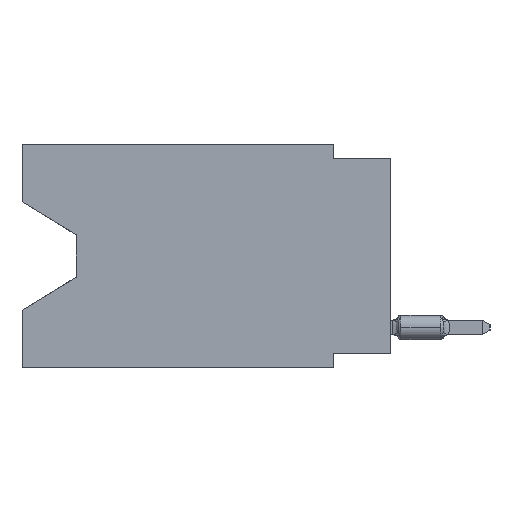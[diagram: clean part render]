
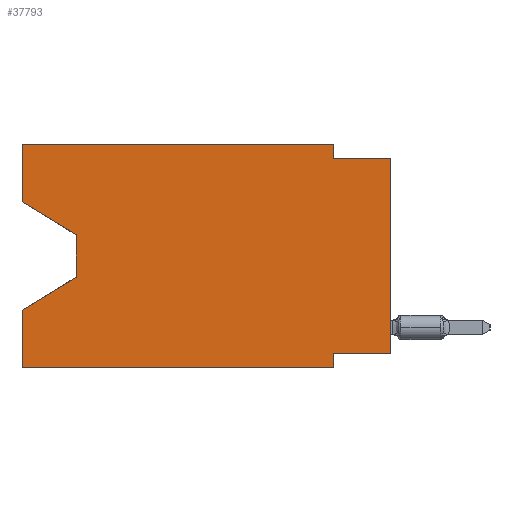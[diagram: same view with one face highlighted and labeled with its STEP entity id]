
A CAD part, left-side view. The second image highlights one B-rep face of the part: STEP entity #37793.
In plain terms, the highlighted planar face has unit normal (-1, 0, 0).
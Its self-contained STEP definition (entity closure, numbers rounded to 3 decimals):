
#69 = VERTEX_POINT ( 'NONE', #26142 ) ;
#154 = ORIENTED_EDGE ( 'NONE', *, *, #14962, .F. ) ;
#1042 = VERTEX_POINT ( 'NONE', #56922 ) ;
#2557 = DIRECTION ( 'NONE',  ( 0., 0.855, -0.519 ) ) ;
#2766 = VECTOR ( 'NONE', #8453, 1000. ) ;
#2847 = DIRECTION ( 'NONE',  ( 0., -1., 0. ) ) ;
#4312 = VERTEX_POINT ( 'NONE', #74643 ) ;
#6569 = LINE ( 'NONE', #58709, #25893 ) ;
#6645 = LINE ( 'NONE', #53426, #15274 ) ;
#7734 = DIRECTION ( 'NONE',  ( 0., 0., -1. ) ) ;
#8318 = LINE ( 'NONE', #25927, #33434 ) ;
#8453 = DIRECTION ( 'NONE',  ( 0., 0., -1. ) ) ;
#9292 = ORIENTED_EDGE ( 'NONE', *, *, #17592, .T. ) ;
#9833 = CARTESIAN_POINT ( 'NONE',  ( 0., 2.54, -9.906 ) ) ;
#10333 = LINE ( 'NONE', #52889, #56960 ) ;
#10784 = CARTESIAN_POINT ( 'NONE',  ( 0., 2.54, 0. ) ) ;
#10847 = CARTESIAN_POINT ( 'NONE',  ( 0., 2.54, 0. ) ) ;
#12962 = DIRECTION ( 'NONE',  ( 0., 0., -1. ) ) ;
#13139 = DIRECTION ( 'NONE',  ( 0., 0., -1. ) ) ;
#13227 = CARTESIAN_POINT ( 'NONE',  ( 0., 13.97, -4.013 ) ) ;
#14686 = AXIS2_PLACEMENT_3D ( 'NONE', #66761, #37614, #13139 ) ;
#14962 = EDGE_CURVE ( 'NONE', #1042, #27319, #39670, .T. ) ;
#15274 = VECTOR ( 'NONE', #18509, 1000. ) ;
#17400 = CARTESIAN_POINT ( 'NONE',  ( 0., 16.383, -2.546 ) ) ;
#17592 = EDGE_CURVE ( 'NONE', #47912, #22956, #18839, .T. ) ;
#18509 = DIRECTION ( 'NONE',  ( 0., 1., 0. ) ) ;
#18839 = LINE ( 'NONE', #60257, #19649 ) ;
#19649 = VECTOR ( 'NONE', #7734, 1000. ) ;
#20201 = ORIENTED_EDGE ( 'NONE', *, *, #43544, .F. ) ;
#20204 = EDGE_CURVE ( 'NONE', #65862, #1042, #6569, .T. ) ;
#20743 = FACE_OUTER_BOUND ( 'NONE', #42780, .T. ) ;
#22283 = DIRECTION ( 'NONE',  ( 0., 0., 1. ) ) ;
#22810 = VERTEX_POINT ( 'NONE', #56799 ) ;
#22956 = VERTEX_POINT ( 'NONE', #27642 ) ;
#23275 = ORIENTED_EDGE ( 'NONE', *, *, #66403, .F. ) ;
#23717 = EDGE_CURVE ( 'NONE', #22956, #34299, #8318, .T. ) ;
#25504 = VECTOR ( 'NONE', #57700, 1000. ) ;
#25619 = EDGE_CURVE ( 'NONE', #22810, #41762, #6645, .T. ) ;
#25893 = VECTOR ( 'NONE', #22283, 1000. ) ;
#25927 = CARTESIAN_POINT ( 'NONE',  ( 0., 13.97, -5.893 ) ) ;
#26142 = CARTESIAN_POINT ( 'NONE',  ( 0., 0., -0.635 ) ) ;
#26453 = CARTESIAN_POINT ( 'NONE',  ( 0., 2.54, -9.906 ) ) ;
#27319 = VERTEX_POINT ( 'NONE', #10847 ) ;
#27642 = CARTESIAN_POINT ( 'NONE',  ( 0., 13.97, -5.893 ) ) ;
#28023 = ORIENTED_EDGE ( 'NONE', *, *, #20204, .F. ) ;
#28178 = LINE ( 'NONE', #33178, #43076 ) ;
#28193 = VECTOR ( 'NONE', #28244, 1000. ) ;
#28244 = DIRECTION ( 'NONE',  ( 0., -0.855, -0.519 ) ) ;
#29385 = CARTESIAN_POINT ( 'NONE',  ( 0., 16.383, -2.546 ) ) ;
#30999 = VERTEX_POINT ( 'NONE', #74027 ) ;
#32113 = ORIENTED_EDGE ( 'NONE', *, *, #50423, .T. ) ;
#32631 = DIRECTION ( 'NONE',  ( 0., 0., 1. ) ) ;
#33057 = VERTEX_POINT ( 'NONE', #9833 ) ;
#33178 = CARTESIAN_POINT ( 'NONE',  ( 0., 16.383, -9.906 ) ) ;
#33434 = VECTOR ( 'NONE', #2557, 1000. ) ;
#33572 = VECTOR ( 'NONE', #12962, 1000. ) ;
#34106 = ORIENTED_EDGE ( 'NONE', *, *, #59403, .F. ) ;
#34299 = VERTEX_POINT ( 'NONE', #51605 ) ;
#34538 = LINE ( 'NONE', #10784, #33572 ) ;
#34739 = LINE ( 'NONE', #29385, #28193 ) ;
#36752 = EDGE_CURVE ( 'NONE', #4312, #34299, #61768, .T. ) ;
#37614 = DIRECTION ( 'NONE',  ( 1., 0., 0. ) ) ;
#37793 = ADVANCED_FACE ( 'NONE', ( #20743 ), #44136, .F. ) ;
#39302 = DIRECTION ( 'NONE',  ( 0., -1., 0. ) ) ;
#39670 = LINE ( 'NONE', #75320, #25504 ) ;
#41762 = VERTEX_POINT ( 'NONE', #55363 ) ;
#42780 = EDGE_LOOP ( 'NONE', ( #43216, #9292, #49295, #65210, #62398, #23275, #44096, #32113, #34106, #20201, #154, #28023 ) ) ;
#43076 = VECTOR ( 'NONE', #39302, 1000. ) ;
#43216 = ORIENTED_EDGE ( 'NONE', *, *, #65258, .T. ) ;
#43544 = EDGE_CURVE ( 'NONE', #27319, #30999, #34538, .T. ) ;
#44096 = ORIENTED_EDGE ( 'NONE', *, *, #25619, .F. ) ;
#44136 = PLANE ( 'NONE',  #14686 ) ;
#47912 = VERTEX_POINT ( 'NONE', #13227 ) ;
#48189 = CARTESIAN_POINT ( 'NONE',  ( 0., 0., -0.635 ) ) ;
#49295 = ORIENTED_EDGE ( 'NONE', *, *, #23717, .T. ) ;
#50423 = EDGE_CURVE ( 'NONE', #22810, #69, #10333, .T. ) ;
#51605 = CARTESIAN_POINT ( 'NONE',  ( 0., 16.383, -7.36 ) ) ;
#52110 = DIRECTION ( 'NONE',  ( 0., 0., 1. ) ) ;
#52889 = CARTESIAN_POINT ( 'NONE',  ( 0., 0., 0. ) ) ;
#53426 = CARTESIAN_POINT ( 'NONE',  ( 0., 0., -9.271 ) ) ;
#55363 = CARTESIAN_POINT ( 'NONE',  ( 0., 2.54, -9.271 ) ) ;
#55642 = CARTESIAN_POINT ( 'NONE',  ( 0., 16.383, 0. ) ) ;
#56799 = CARTESIAN_POINT ( 'NONE',  ( 0., 0., -9.271 ) ) ;
#56922 = CARTESIAN_POINT ( 'NONE',  ( 0., 16.383, 0. ) ) ;
#56960 = VECTOR ( 'NONE', #52110, 1000. ) ;
#57700 = DIRECTION ( 'NONE',  ( 0., -1., 0. ) ) ;
#58709 = CARTESIAN_POINT ( 'NONE',  ( 0., 16.383, 0. ) ) ;
#59403 = EDGE_CURVE ( 'NONE', #30999, #69, #65826, .T. ) ;
#60227 = LINE ( 'NONE', #26453, #2766 ) ;
#60257 = CARTESIAN_POINT ( 'NONE',  ( 0., 13.97, -4.013 ) ) ;
#61768 = LINE ( 'NONE', #55642, #68448 ) ;
#62398 = ORIENTED_EDGE ( 'NONE', *, *, #67337, .T. ) ;
#65210 = ORIENTED_EDGE ( 'NONE', *, *, #36752, .F. ) ;
#65258 = EDGE_CURVE ( 'NONE', #65862, #47912, #34739, .T. ) ;
#65826 = LINE ( 'NONE', #48189, #70515 ) ;
#65862 = VERTEX_POINT ( 'NONE', #17400 ) ;
#66403 = EDGE_CURVE ( 'NONE', #41762, #33057, #60227, .T. ) ;
#66761 = CARTESIAN_POINT ( 'NONE',  ( 0., 16.383, 0. ) ) ;
#67337 = EDGE_CURVE ( 'NONE', #4312, #33057, #28178, .T. ) ;
#68448 = VECTOR ( 'NONE', #32631, 1000. ) ;
#70515 = VECTOR ( 'NONE', #2847, 1000. ) ;
#74027 = CARTESIAN_POINT ( 'NONE',  ( 0., 2.54, -0.635 ) ) ;
#74643 = CARTESIAN_POINT ( 'NONE',  ( 0., 16.383, -9.906 ) ) ;
#75320 = CARTESIAN_POINT ( 'NONE',  ( 0., 16.383, 0. ) ) ;
